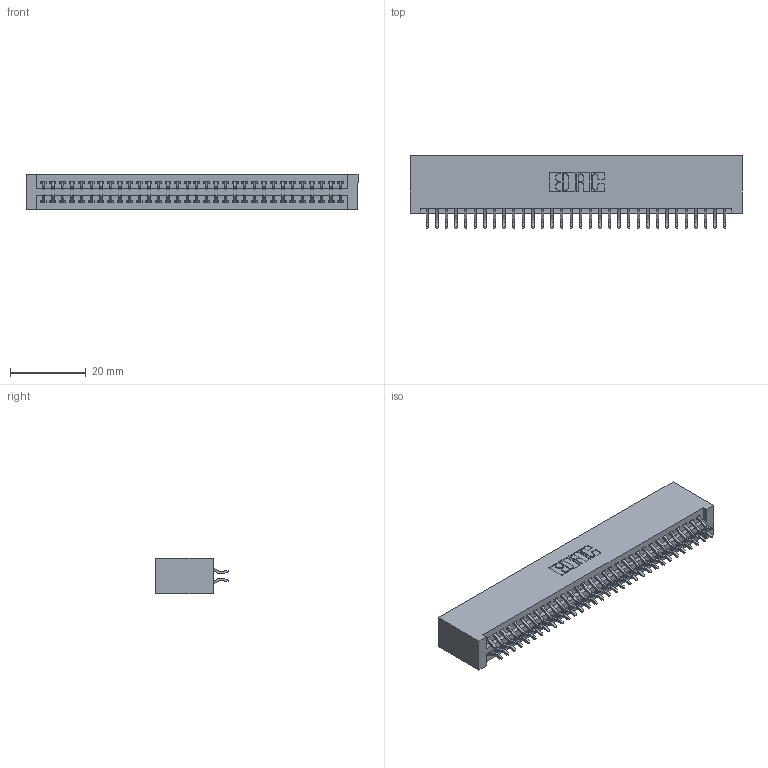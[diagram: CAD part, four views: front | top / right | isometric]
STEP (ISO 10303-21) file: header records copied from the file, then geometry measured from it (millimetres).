
FILE_DESCRIPTION (( 'STEP AP203' ), '1' );
FILE_NAME ('395-064-556-201.STEP', '2019-10-23T19:14:57', ( '' ), ( '' ), 'SwSTEP 2.0', 'SolidWorks 2016', '' );
FILE_SCHEMA (( 'CONFIG_CONTROL_DESIGN' ));
Length unit declared in the file: inch
Products named in the file (3): 345-292-001_556 Tail; 395-064-556-201; 345 Part_No Mounting Lugs
Assembly tree (65 placements, depth 2):
  395-064-556-201
    345 Part_No Mounting Lugs
    345-292-001_556 Tail  x64
Bounding box: 87.88 x 19.24 x 9.4 mm (x, y, z)
Volume: 9057.7 mm3; surface area: 13442.4 mm2
Topology: 65 solids, 65 shells, 3702 faces, 11005 edges, 7250 vertices
Faces by surface type: plane 2444, cylinder 1258
Entity records: 26397 total; most frequent: CARTESIAN_POINT 4448, ORIENTED_EDGE 4370, DIRECTION 3917, EDGE_CURVE 2185, VECTOR 1925, LINE 1925, VERTEX_POINT 1454, AXIS2_PLACEMENT_3D 996
